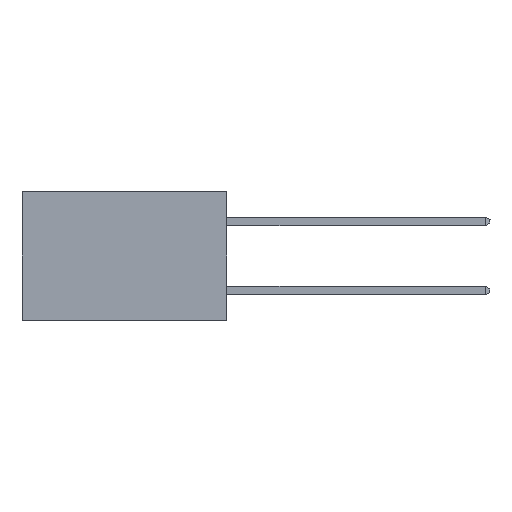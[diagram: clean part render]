
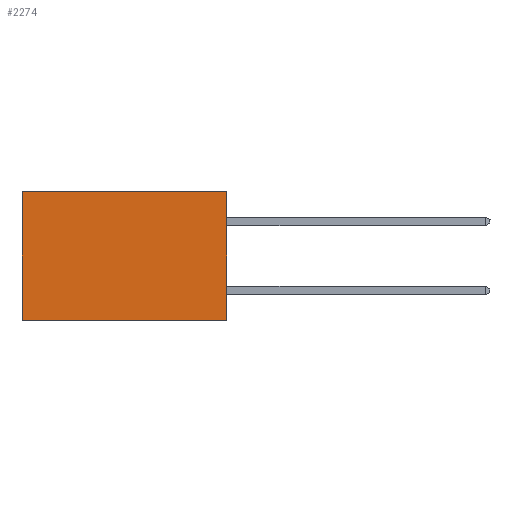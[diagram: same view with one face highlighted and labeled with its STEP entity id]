
A CAD part, left-side view. The second image highlights one B-rep face of the part: STEP entity #2274.
In plain terms, the highlighted planar face has unit normal (-1, 0, 0).
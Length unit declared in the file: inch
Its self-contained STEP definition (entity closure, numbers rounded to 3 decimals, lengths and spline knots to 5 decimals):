
#303 = CARTESIAN_POINT ( 'NONE',  ( 0.277, 0., -0.37 ) ) ;
#1097 = DIRECTION ( 'NONE',  ( 0., 0., -1. ) ) ;
#1315 = CARTESIAN_POINT ( 'NONE',  ( 0.277, 0., -0.37 ) ) ;
#1766 = LINE ( 'NONE', #5293, #3337 ) ;
#1885 = VERTEX_POINT ( 'NONE', #5511 ) ;
#1935 = VERTEX_POINT ( 'NONE', #4376 ) ;
#2173 = EDGE_CURVE ( 'NONE', #2915, #4097, #6240, .T. ) ;
#2274 = ADVANCED_FACE ( 'NONE', ( #4864 ), #6830, .F. ) ;
#2827 = LINE ( 'NONE', #5364, #3873 ) ;
#2915 = VERTEX_POINT ( 'NONE', #303 ) ;
#3073 = EDGE_LOOP ( 'NONE', ( #4801, #4896, #4992, #5184 ) ) ;
#3183 = VECTOR ( 'NONE', #7621, 39.37008 ) ;
#3337 = VECTOR ( 'NONE', #5320, 39.37008 ) ;
#3345 = EDGE_CURVE ( 'NONE', #1935, #1885, #1766, .T. ) ;
#3516 = EDGE_CURVE ( 'NONE', #1935, #2915, #6841, .T. ) ;
#3599 = CARTESIAN_POINT ( 'NONE',  ( 0.277, 0., -0.37 ) ) ;
#3873 = VECTOR ( 'NONE', #5341, 39.37008 ) ;
#4097 = VERTEX_POINT ( 'NONE', #6920 ) ;
#4376 = CARTESIAN_POINT ( 'NONE',  ( 0.277, 0., 0. ) ) ;
#4531 = AXIS2_PLACEMENT_3D ( 'NONE', #6938, #6744, #6731 ) ;
#4621 = EDGE_CURVE ( 'NONE', #1885, #4097, #2827, .T. ) ;
#4801 = ORIENTED_EDGE ( 'NONE', *, *, #4621, .T. ) ;
#4864 = FACE_OUTER_BOUND ( 'NONE', #3073, .T. ) ;
#4896 = ORIENTED_EDGE ( 'NONE', *, *, #2173, .F. ) ;
#4992 = ORIENTED_EDGE ( 'NONE', *, *, #3516, .F. ) ;
#5184 = ORIENTED_EDGE ( 'NONE', *, *, #3345, .T. ) ;
#5218 = VECTOR ( 'NONE', #1097, 39.37008 ) ;
#5293 = CARTESIAN_POINT ( 'NONE',  ( 0.277, 0., 0. ) ) ;
#5320 = DIRECTION ( 'NONE',  ( 0., 1., 0. ) ) ;
#5341 = DIRECTION ( 'NONE',  ( 0., 0., -1. ) ) ;
#5364 = CARTESIAN_POINT ( 'NONE',  ( 0.277, 0.59, -0.37 ) ) ;
#5511 = CARTESIAN_POINT ( 'NONE',  ( 0.277, 0.59, 0. ) ) ;
#6240 = LINE ( 'NONE', #1315, #3183 ) ;
#6731 = DIRECTION ( 'NONE',  ( 0., 0., -1. ) ) ;
#6744 = DIRECTION ( 'NONE',  ( 1., 0., 0. ) ) ;
#6830 = PLANE ( 'NONE',  #4531 ) ;
#6841 = LINE ( 'NONE', #3599, #5218 ) ;
#6920 = CARTESIAN_POINT ( 'NONE',  ( 0.277, 0.59, -0.37 ) ) ;
#6938 = CARTESIAN_POINT ( 'NONE',  ( 0.277, 0., -0.37 ) ) ;
#7621 = DIRECTION ( 'NONE',  ( 0., 1., 0. ) ) ;
